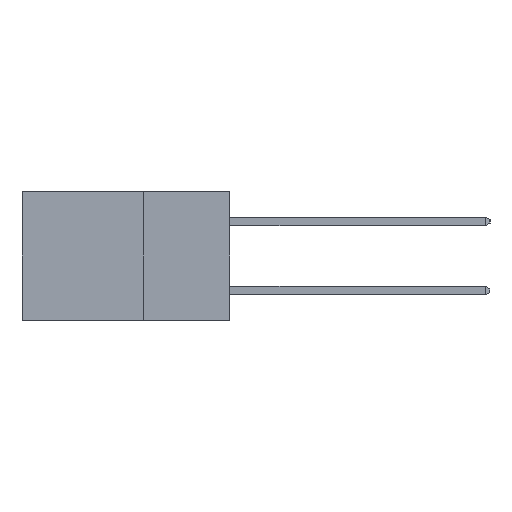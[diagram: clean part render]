
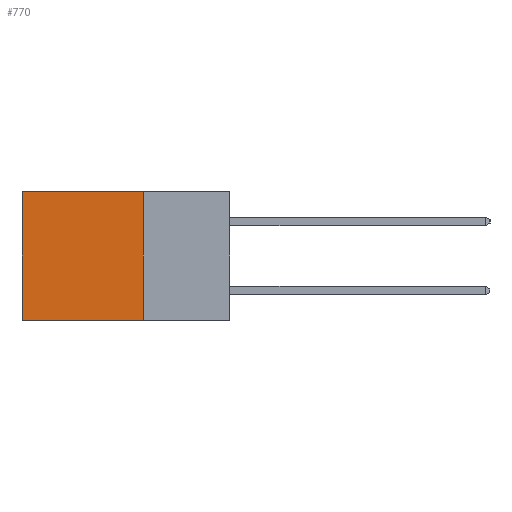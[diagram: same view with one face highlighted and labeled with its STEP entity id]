
A CAD part, left-side view. The second image highlights one B-rep face of the part: STEP entity #770.
In plain terms, the highlighted planar face has unit normal (-1, 0, 0).
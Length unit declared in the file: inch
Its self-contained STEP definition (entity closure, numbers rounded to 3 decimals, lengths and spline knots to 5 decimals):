
#4 = CARTESIAN_POINT ( 'NONE',  ( 0.298, 0.6, 0. ) ) ;
#574 = VECTOR ( 'NONE', #5339, 39.37008 ) ;
#770 = ADVANCED_FACE ( 'NONE', ( #14958 ), #4309, .F. ) ;
#813 = VERTEX_POINT ( 'NONE', #6532 ) ;
#1042 = ORIENTED_EDGE ( 'NONE', *, *, #6217, .T. ) ;
#1278 = EDGE_LOOP ( 'NONE', ( #9978, #8109, #13463, #1042 ) ) ;
#1452 = CARTESIAN_POINT ( 'NONE',  ( 0.298, 0.25, 0. ) ) ;
#1527 = CARTESIAN_POINT ( 'NONE',  ( 0.298, 0.25, 0. ) ) ;
#1583 = AXIS2_PLACEMENT_3D ( 'NONE', #13769, #11869, #4242 ) ;
#4032 = CARTESIAN_POINT ( 'NONE',  ( 0.298, 0.25, -0.37 ) ) ;
#4063 = LINE ( 'NONE', #5289, #574 ) ;
#4242 = DIRECTION ( 'NONE',  ( 0., 0., -1. ) ) ;
#4309 = PLANE ( 'NONE',  #1583 ) ;
#5289 = CARTESIAN_POINT ( 'NONE',  ( 0.298, 0.25, 0. ) ) ;
#5339 = DIRECTION ( 'NONE',  ( 0., 1., 0. ) ) ;
#6217 = EDGE_CURVE ( 'NONE', #13870, #813, #4063, .T. ) ;
#6422 = LINE ( 'NONE', #4, #15763 ) ;
#6532 = CARTESIAN_POINT ( 'NONE',  ( 0.298, 0.6, 0. ) ) ;
#6620 = DIRECTION ( 'NONE',  ( 0., 1., 0. ) ) ;
#6630 = VECTOR ( 'NONE', #15160, 39.37008 ) ;
#6709 = EDGE_CURVE ( 'NONE', #13870, #13152, #9966, .T. ) ;
#6761 = DIRECTION ( 'NONE',  ( 0., 0., -1. ) ) ;
#7161 = VECTOR ( 'NONE', #6620, 39.37008 ) ;
#7916 = VERTEX_POINT ( 'NONE', #12423 ) ;
#8109 = ORIENTED_EDGE ( 'NONE', *, *, #13834, .F. ) ;
#9966 = LINE ( 'NONE', #1452, #6630 ) ;
#9978 = ORIENTED_EDGE ( 'NONE', *, *, #12605, .T. ) ;
#10466 = LINE ( 'NONE', #11520, #7161 ) ;
#11520 = CARTESIAN_POINT ( 'NONE',  ( 0.298, 0.25, -0.37 ) ) ;
#11869 = DIRECTION ( 'NONE',  ( 1., 0., 0. ) ) ;
#12423 = CARTESIAN_POINT ( 'NONE',  ( 0.298, 0.6, -0.37 ) ) ;
#12605 = EDGE_CURVE ( 'NONE', #813, #7916, #6422, .T. ) ;
#13152 = VERTEX_POINT ( 'NONE', #4032 ) ;
#13463 = ORIENTED_EDGE ( 'NONE', *, *, #6709, .F. ) ;
#13769 = CARTESIAN_POINT ( 'NONE',  ( 0.298, 0.25, 0. ) ) ;
#13834 = EDGE_CURVE ( 'NONE', #13152, #7916, #10466, .T. ) ;
#13870 = VERTEX_POINT ( 'NONE', #1527 ) ;
#14958 = FACE_OUTER_BOUND ( 'NONE', #1278, .T. ) ;
#15160 = DIRECTION ( 'NONE',  ( 0., 0., -1. ) ) ;
#15763 = VECTOR ( 'NONE', #6761, 39.37008 ) ;
